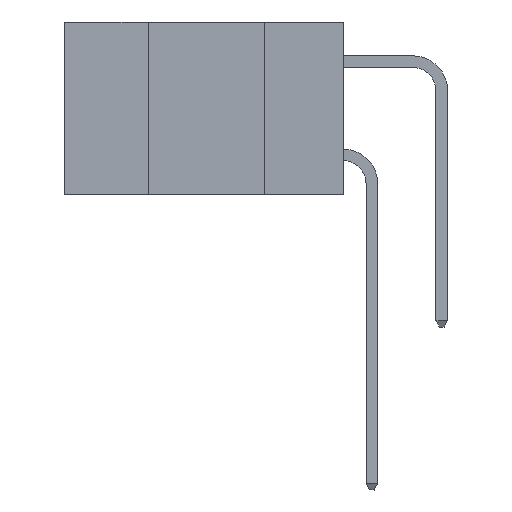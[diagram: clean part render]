
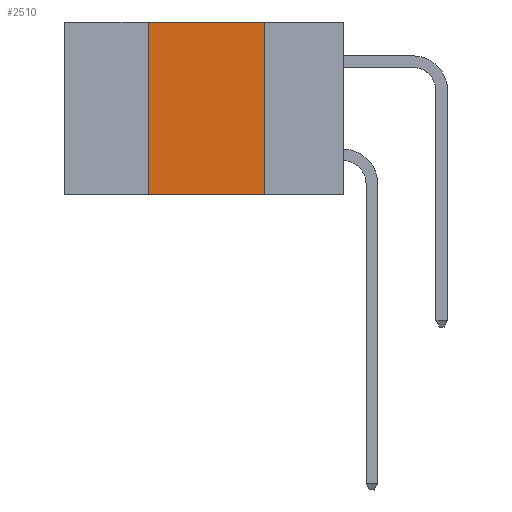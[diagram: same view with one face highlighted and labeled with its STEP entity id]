
A CAD part, left-side view. The second image highlights one B-rep face of the part: STEP entity #2510.
In plain terms, the highlighted planar face has unit normal (-1, 0, 0).
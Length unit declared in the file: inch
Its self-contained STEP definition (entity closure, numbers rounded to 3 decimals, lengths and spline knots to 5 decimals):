
#1813 = VERTEX_POINT ( 'NONE', #11640 ) ;
#1858 = CARTESIAN_POINT ( 'NONE',  ( 0., 0.6, -0.37 ) ) ;
#2242 = EDGE_CURVE ( 'NONE', #15567, #12024, #16159, .T. ) ;
#2336 = CARTESIAN_POINT ( 'NONE',  ( 0., 0.17, -0.37 ) ) ;
#2510 = ADVANCED_FACE ( 'NONE', ( #2636 ), #17829, .F. ) ;
#2584 = EDGE_CURVE ( 'NONE', #1813, #15567, #6453, .T. ) ;
#2636 = FACE_OUTER_BOUND ( 'NONE', #16167, .T. ) ;
#3185 = DIRECTION ( 'NONE',  ( 0., 0., -1. ) ) ;
#3762 = DIRECTION ( 'NONE',  ( 0., 0., 1. ) ) ;
#4310 = ORIENTED_EDGE ( 'NONE', *, *, #2584, .F. ) ;
#6077 = LINE ( 'NONE', #13242, #13763 ) ;
#6092 = EDGE_CURVE ( 'NONE', #12024, #13558, #6077, .T. ) ;
#6422 = DIRECTION ( 'NONE',  ( 0., -1., 0. ) ) ;
#6453 = LINE ( 'NONE', #12067, #13797 ) ;
#7518 = DIRECTION ( 'NONE',  ( 0., -1., 0. ) ) ;
#8122 = DIRECTION ( 'NONE',  ( 0., 0., -1. ) ) ;
#8481 = EDGE_CURVE ( 'NONE', #1813, #13558, #16166, .T. ) ;
#8742 = ORIENTED_EDGE ( 'NONE', *, *, #8481, .T. ) ;
#11105 = CARTESIAN_POINT ( 'NONE',  ( 0., 0.42, 0. ) ) ;
#11640 = CARTESIAN_POINT ( 'NONE',  ( 0., 0.42, -0.37 ) ) ;
#12024 = VERTEX_POINT ( 'NONE', #12074 ) ;
#12067 = CARTESIAN_POINT ( 'NONE',  ( 0., 0.42, -0.37 ) ) ;
#12074 = CARTESIAN_POINT ( 'NONE',  ( 0., 0.17, 0. ) ) ;
#13242 = CARTESIAN_POINT ( 'NONE',  ( 0., 0.17, -0.37 ) ) ;
#13372 = AXIS2_PLACEMENT_3D ( 'NONE', #15161, #13516, #8122 ) ;
#13386 = CARTESIAN_POINT ( 'NONE',  ( 0., 0.6, 0. ) ) ;
#13457 = VECTOR ( 'NONE', #7518, 39.37008 ) ;
#13516 = DIRECTION ( 'NONE',  ( 1., 0., 0. ) ) ;
#13558 = VERTEX_POINT ( 'NONE', #2336 ) ;
#13763 = VECTOR ( 'NONE', #3185, 39.37008 ) ;
#13797 = VECTOR ( 'NONE', #3762, 39.37008 ) ;
#14827 = ORIENTED_EDGE ( 'NONE', *, *, #2242, .F. ) ;
#15161 = CARTESIAN_POINT ( 'NONE',  ( 0., 0.6, 0. ) ) ;
#15567 = VERTEX_POINT ( 'NONE', #11105 ) ;
#15775 = ORIENTED_EDGE ( 'NONE', *, *, #6092, .F. ) ;
#16159 = LINE ( 'NONE', #13386, #16865 ) ;
#16166 = LINE ( 'NONE', #1858, #13457 ) ;
#16167 = EDGE_LOOP ( 'NONE', ( #15775, #14827, #4310, #8742 ) ) ;
#16865 = VECTOR ( 'NONE', #6422, 39.37008 ) ;
#17829 = PLANE ( 'NONE',  #13372 ) ;
